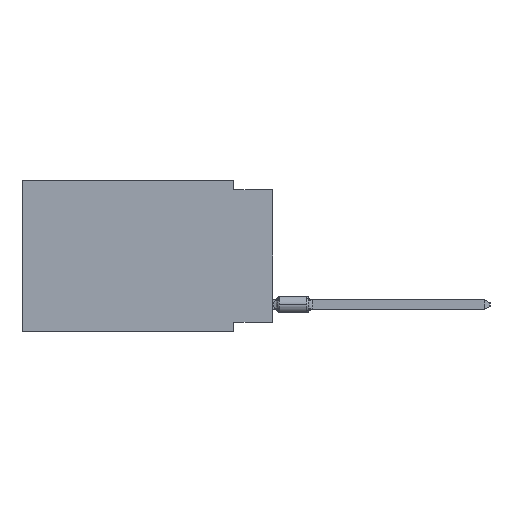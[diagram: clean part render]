
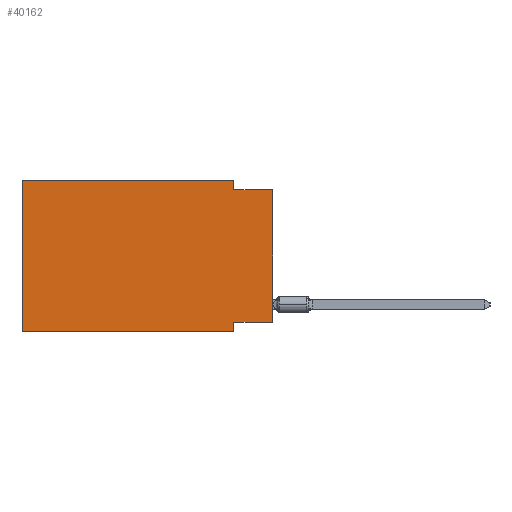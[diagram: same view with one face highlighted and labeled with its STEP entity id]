
A CAD part, left-side view. The second image highlights one B-rep face of the part: STEP entity #40162.
In plain terms, the highlighted planar face has unit normal (-1, 0, 0).
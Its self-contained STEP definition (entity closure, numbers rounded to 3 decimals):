
#907 = EDGE_CURVE ( 'NONE', #36456, #36187, #39731, .T. ) ;
#2148 = LINE ( 'NONE', #28631, #27671 ) ;
#2499 = EDGE_CURVE ( 'NONE', #3473, #30367, #2148, .T. ) ;
#2594 = PLANE ( 'NONE',  #24334 ) ;
#3473 = VERTEX_POINT ( 'NONE', #27833 ) ;
#3522 = ORIENTED_EDGE ( 'NONE', *, *, #19758, .F. ) ;
#3612 = VECTOR ( 'NONE', #36745, 1000. ) ;
#3631 = CARTESIAN_POINT ( 'NONE',  ( 0., 0., -0.635 ) ) ;
#4775 = DIRECTION ( 'NONE',  ( 0., 0., -1. ) ) ;
#5531 = CARTESIAN_POINT ( 'NONE',  ( 0., 16.383, 0. ) ) ;
#5714 = VERTEX_POINT ( 'NONE', #12267 ) ;
#5860 = DIRECTION ( 'NONE',  ( 1., 0., 0. ) ) ;
#8246 = LINE ( 'NONE', #30451, #3612 ) ;
#8516 = VECTOR ( 'NONE', #14124, 1000. ) ;
#10917 = DIRECTION ( 'NONE',  ( 0., 0., -1. ) ) ;
#11499 = EDGE_CURVE ( 'NONE', #26505, #28254, #41309, .T. ) ;
#12267 = CARTESIAN_POINT ( 'NONE',  ( 0., 0., -9.271 ) ) ;
#12285 = ORIENTED_EDGE ( 'NONE', *, *, #33770, .F. ) ;
#12510 = CARTESIAN_POINT ( 'NONE',  ( 0., 2.54, -9.906 ) ) ;
#12808 = VECTOR ( 'NONE', #10917, 1000. ) ;
#13040 = LINE ( 'NONE', #26273, #40189 ) ;
#13419 = EDGE_CURVE ( 'NONE', #5714, #35856, #37426, .T. ) ;
#14124 = DIRECTION ( 'NONE',  ( 0., -1., 0. ) ) ;
#14634 = CARTESIAN_POINT ( 'NONE',  ( 0., 0., 0. ) ) ;
#14866 = ORIENTED_EDGE ( 'NONE', *, *, #2499, .F. ) ;
#18041 = ORIENTED_EDGE ( 'NONE', *, *, #13419, .T. ) ;
#18290 = ORIENTED_EDGE ( 'NONE', *, *, #37240, .T. ) ;
#19097 = FACE_OUTER_BOUND ( 'NONE', #30213, .T. ) ;
#19758 = EDGE_CURVE ( 'NONE', #36187, #26505, #24556, .T. ) ;
#20345 = VECTOR ( 'NONE', #36439, 1000. ) ;
#20679 = CARTESIAN_POINT ( 'NONE',  ( 0., 2.54, 0. ) ) ;
#21455 = VECTOR ( 'NONE', #37873, 1000. ) ;
#24334 = AXIS2_PLACEMENT_3D ( 'NONE', #25391, #5860, #28226 ) ;
#24429 = ORIENTED_EDGE ( 'NONE', *, *, #31210, .F. ) ;
#24556 = LINE ( 'NONE', #37972, #8516 ) ;
#25391 = CARTESIAN_POINT ( 'NONE',  ( 0., 16.383, 0. ) ) ;
#26273 = CARTESIAN_POINT ( 'NONE',  ( 0., 0., -9.271 ) ) ;
#26505 = VERTEX_POINT ( 'NONE', #29765 ) ;
#27330 = LINE ( 'NONE', #33645, #20345 ) ;
#27671 = VECTOR ( 'NONE', #4775, 1000. ) ;
#27833 = CARTESIAN_POINT ( 'NONE',  ( 0., 2.54, -9.271 ) ) ;
#28226 = DIRECTION ( 'NONE',  ( 0., 0., -1. ) ) ;
#28254 = VERTEX_POINT ( 'NONE', #40835 ) ;
#28631 = CARTESIAN_POINT ( 'NONE',  ( 0., 2.54, -9.906 ) ) ;
#29765 = CARTESIAN_POINT ( 'NONE',  ( 0., 2.54, 0. ) ) ;
#30213 = EDGE_LOOP ( 'NONE', ( #18041, #12285, #37001, #3522, #36010, #18290, #14866, #24429 ) ) ;
#30367 = VERTEX_POINT ( 'NONE', #12510 ) ;
#30451 = CARTESIAN_POINT ( 'NONE',  ( 0., 0., -0.635 ) ) ;
#31210 = EDGE_CURVE ( 'NONE', #5714, #3473, #13040, .T. ) ;
#33246 = DIRECTION ( 'NONE',  ( 0., 1., 0. ) ) ;
#33645 = CARTESIAN_POINT ( 'NONE',  ( 0., 16.383, -9.906 ) ) ;
#33770 = EDGE_CURVE ( 'NONE', #28254, #35856, #8246, .T. ) ;
#35819 = DIRECTION ( 'NONE',  ( 0., 0., 1. ) ) ;
#35856 = VERTEX_POINT ( 'NONE', #3631 ) ;
#36010 = ORIENTED_EDGE ( 'NONE', *, *, #907, .F. ) ;
#36187 = VERTEX_POINT ( 'NONE', #5531 ) ;
#36439 = DIRECTION ( 'NONE',  ( 0., -1., 0. ) ) ;
#36456 = VERTEX_POINT ( 'NONE', #37622 ) ;
#36745 = DIRECTION ( 'NONE',  ( 0., -1., 0. ) ) ;
#37001 = ORIENTED_EDGE ( 'NONE', *, *, #11499, .F. ) ;
#37240 = EDGE_CURVE ( 'NONE', #36456, #30367, #27330, .T. ) ;
#37426 = LINE ( 'NONE', #14634, #21455 ) ;
#37622 = CARTESIAN_POINT ( 'NONE',  ( 0., 16.383, -9.906 ) ) ;
#37873 = DIRECTION ( 'NONE',  ( 0., 0., 1. ) ) ;
#37972 = CARTESIAN_POINT ( 'NONE',  ( 0., 16.383, 0. ) ) ;
#39731 = LINE ( 'NONE', #42558, #40913 ) ;
#40162 = ADVANCED_FACE ( 'NONE', ( #19097 ), #2594, .F. ) ;
#40189 = VECTOR ( 'NONE', #33246, 1000. ) ;
#40835 = CARTESIAN_POINT ( 'NONE',  ( 0., 2.54, -0.635 ) ) ;
#40913 = VECTOR ( 'NONE', #35819, 1000. ) ;
#41309 = LINE ( 'NONE', #20679, #12808 ) ;
#42558 = CARTESIAN_POINT ( 'NONE',  ( 0., 16.383, 0. ) ) ;
